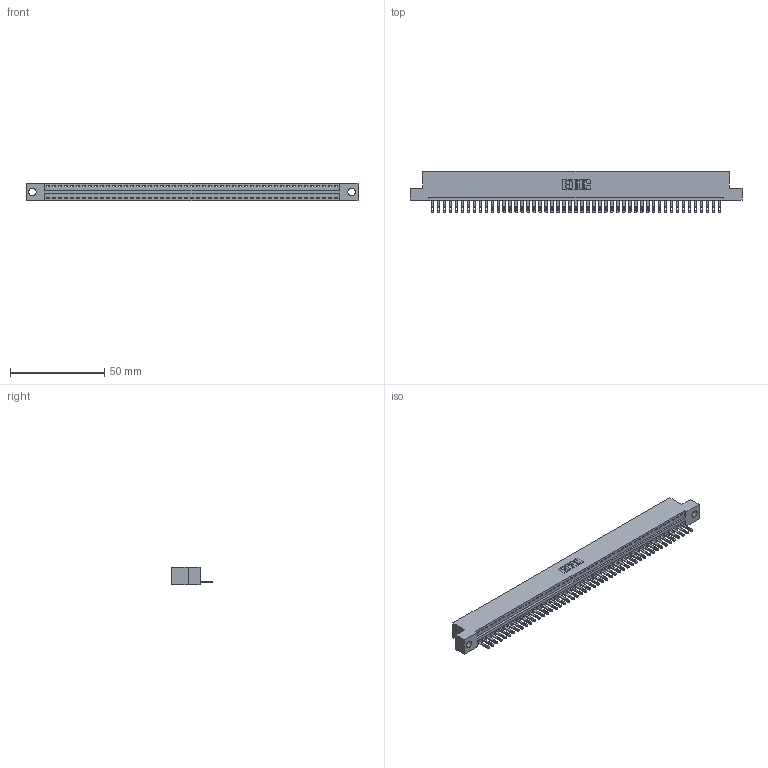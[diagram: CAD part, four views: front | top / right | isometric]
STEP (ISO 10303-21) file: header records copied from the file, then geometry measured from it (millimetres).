
FILE_DESCRIPTION (( 'STEP AP203' ), '1' );
FILE_NAME ('896-049-500-104.STEP', '2021-07-27T23:14:39', ( '' ), ( '' ), 'SwSTEP 2.0', 'SolidWorks 2020', '' );
FILE_SCHEMA (( 'CONFIG_CONTROL_DESIGN' ));
Length unit declared in the file: inch
Products named in the file (3): 896-049-500-104; 345-292-001_345-293-100; 846 Part_Flush Mounting Lugs - 0.156 Dia-TH
Assembly tree (50 placements, depth 2):
  896-049-500-104
    846 Part_Flush Mounting Lugs - 0.156 Dia-TH
    345-292-001_345-293-100  x49
Bounding box: 176.15 x 21.84 x 9.4 mm (x, y, z)
Volume: 16852.1 mm3; surface area: 21057.6 mm2
Topology: 50 solids, 50 shells, 2768 faces, 8561 edges, 5706 vertices
Faces by surface type: plane 1742, cylinder 1026
Entity records: 29401 total; most frequent: CARTESIAN_POINT 5043, ORIENTED_EDGE 5026, DIRECTION 4443, EDGE_CURVE 2513, VECTOR 2181, LINE 2181, VERTEX_POINT 1674, AXIS2_PLACEMENT_3D 1131
